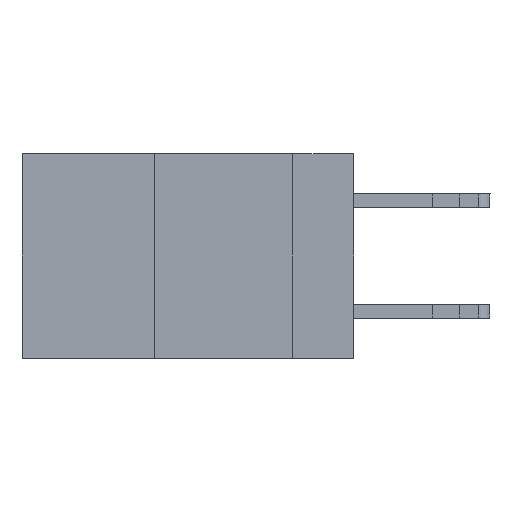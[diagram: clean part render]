
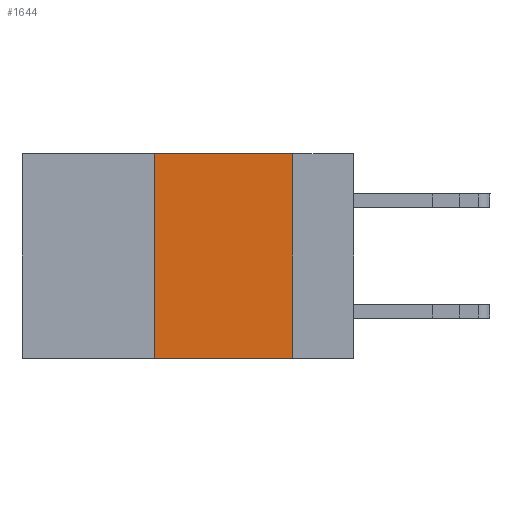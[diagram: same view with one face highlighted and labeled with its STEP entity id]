
A CAD part, left-side view. The second image highlights one B-rep face of the part: STEP entity #1644.
In plain terms, the highlighted planar face has unit normal (-1, 0, 0).
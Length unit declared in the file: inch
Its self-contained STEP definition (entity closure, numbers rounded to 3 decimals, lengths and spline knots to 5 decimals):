
#60 = VERTEX_POINT ( 'NONE', #8732 ) ;
#895 = LINE ( 'NONE', #5276, #5952 ) ;
#1228 = LINE ( 'NONE', #11627, #18709 ) ;
#1516 = ORIENTED_EDGE ( 'NONE', *, *, #3568, .F. ) ;
#1644 = ADVANCED_FACE ( 'NONE', ( #8328 ), #18412, .F. ) ;
#2273 = VECTOR ( 'NONE', #17830, 39.37008 ) ;
#3568 = EDGE_CURVE ( 'NONE', #60, #7418, #1228, .T. ) ;
#3760 = DIRECTION ( 'NONE',  ( 1., 0., 0. ) ) ;
#3956 = CARTESIAN_POINT ( 'NONE',  ( 0., 0.11, -0.37 ) ) ;
#3957 = CARTESIAN_POINT ( 'NONE',  ( 0., 0.6, 0. ) ) ;
#4907 = DIRECTION ( 'NONE',  ( 0., 0., -1. ) ) ;
#5138 = DIRECTION ( 'NONE',  ( 0., 0., -1. ) ) ;
#5276 = CARTESIAN_POINT ( 'NONE',  ( 0., 0.6, -0.37 ) ) ;
#5952 = VECTOR ( 'NONE', #8285, 39.37008 ) ;
#6266 = LINE ( 'NONE', #15378, #15288 ) ;
#7149 = DIRECTION ( 'NONE',  ( 0., -1., 0. ) ) ;
#7418 = VERTEX_POINT ( 'NONE', #9326 ) ;
#8285 = DIRECTION ( 'NONE',  ( 0., -1., 0. ) ) ;
#8328 = FACE_OUTER_BOUND ( 'NONE', #16265, .T. ) ;
#8732 = CARTESIAN_POINT ( 'NONE',  ( 0., 0.36, 0. ) ) ;
#8931 = LINE ( 'NONE', #16568, #2273 ) ;
#8982 = ORIENTED_EDGE ( 'NONE', *, *, #12326, .F. ) ;
#9326 = CARTESIAN_POINT ( 'NONE',  ( 0., 0.11, 0. ) ) ;
#9762 = EDGE_CURVE ( 'NONE', #18271, #60, #8931, .T. ) ;
#9768 = ORIENTED_EDGE ( 'NONE', *, *, #17955, .T. ) ;
#10098 = AXIS2_PLACEMENT_3D ( 'NONE', #3957, #3760, #5138 ) ;
#11627 = CARTESIAN_POINT ( 'NONE',  ( 0., 0.6, 0. ) ) ;
#12326 = EDGE_CURVE ( 'NONE', #7418, #19019, #6266, .T. ) ;
#12551 = ORIENTED_EDGE ( 'NONE', *, *, #9762, .F. ) ;
#15288 = VECTOR ( 'NONE', #4907, 39.37008 ) ;
#15378 = CARTESIAN_POINT ( 'NONE',  ( 0., 0.11, 0. ) ) ;
#16265 = EDGE_LOOP ( 'NONE', ( #8982, #1516, #12551, #9768 ) ) ;
#16568 = CARTESIAN_POINT ( 'NONE',  ( 0., 0.36, 0. ) ) ;
#16589 = CARTESIAN_POINT ( 'NONE',  ( 0., 0.36, -0.37 ) ) ;
#17830 = DIRECTION ( 'NONE',  ( 0., 0., 1. ) ) ;
#17955 = EDGE_CURVE ( 'NONE', #18271, #19019, #895, .T. ) ;
#18271 = VERTEX_POINT ( 'NONE', #16589 ) ;
#18412 = PLANE ( 'NONE',  #10098 ) ;
#18709 = VECTOR ( 'NONE', #7149, 39.37008 ) ;
#19019 = VERTEX_POINT ( 'NONE', #3956 ) ;
